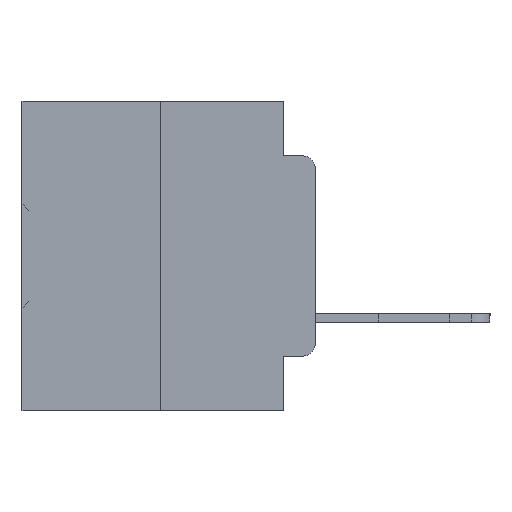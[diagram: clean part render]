
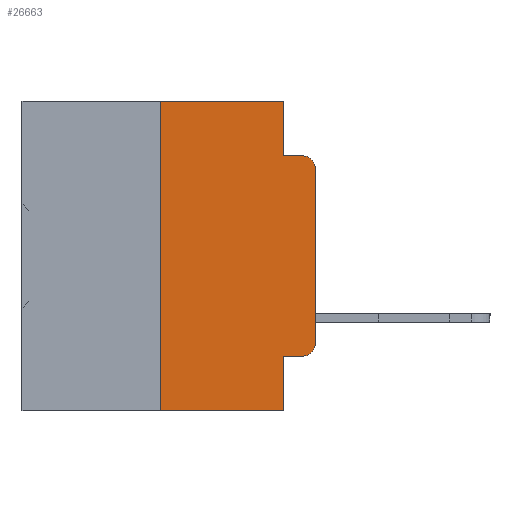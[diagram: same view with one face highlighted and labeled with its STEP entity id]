
A CAD part, left-side view. The second image highlights one B-rep face of the part: STEP entity #26663.
In plain terms, the highlighted planar face has unit normal (-1, 0, 0).
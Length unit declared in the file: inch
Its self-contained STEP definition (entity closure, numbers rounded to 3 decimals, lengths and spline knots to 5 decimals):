
#154 = DIRECTION ( 'NONE',  ( 0., 0., -1. ) ) ;
#941 = FACE_OUTER_BOUND ( 'NONE', #30080, .T. ) ;
#1112 = ORIENTED_EDGE ( 'NONE', *, *, #12248, .T. ) ;
#1768 = VERTEX_POINT ( 'NONE', #36380 ) ;
#2023 = DIRECTION ( 'NONE',  ( 0., 0., -1. ) ) ;
#2344 = LINE ( 'NONE', #2949, #23385 ) ;
#2350 = CARTESIAN_POINT ( 'NONE',  ( 0., 0.02, -0.4115 ) ) ;
#2720 = DIRECTION ( 'NONE',  ( 0., 0., -1. ) ) ;
#2949 = CARTESIAN_POINT ( 'NONE',  ( 0., 0.473, 0. ) ) ;
#2981 = VERTEX_POINT ( 'NONE', #11474 ) ;
#3852 = LINE ( 'NONE', #6824, #25783 ) ;
#5730 = EDGE_CURVE ( 'NONE', #36417, #1768, #3852, .T. ) ;
#5749 = CARTESIAN_POINT ( 'NONE',  ( 0., 0.25, -0.5 ) ) ;
#6105 = ORIENTED_EDGE ( 'NONE', *, *, #5730, .T. ) ;
#6185 = AXIS2_PLACEMENT_3D ( 'NONE', #30549, #13515, #33371 ) ;
#6299 = CARTESIAN_POINT ( 'NONE',  ( 0., 0.25, 0. ) ) ;
#6824 = CARTESIAN_POINT ( 'NONE',  ( 0., 0., 0. ) ) ;
#6929 = VERTEX_POINT ( 'NONE', #24255 ) ;
#7170 = LINE ( 'NONE', #9047, #21484 ) ;
#7693 = CARTESIAN_POINT ( 'NONE',  ( 0., 0.473, 0. ) ) ;
#7795 = CIRCLE ( 'NONE', #6185, 0.02 ) ;
#7893 = VECTOR ( 'NONE', #21350, 39.37008 ) ;
#8385 = CIRCLE ( 'NONE', #18694, 0.02 ) ;
#8658 = ORIENTED_EDGE ( 'NONE', *, *, #14152, .T. ) ;
#9005 = LINE ( 'NONE', #16842, #24184 ) ;
#9047 = CARTESIAN_POINT ( 'NONE',  ( 0., 0.051, -0.0885 ) ) ;
#9092 = DIRECTION ( 'NONE',  ( 0., 0., -1. ) ) ;
#9466 = LINE ( 'NONE', #34334, #23746 ) ;
#10687 = VECTOR ( 'NONE', #9092, 39.37008 ) ;
#11379 = AXIS2_PLACEMENT_3D ( 'NONE', #7693, #19181, #2023 ) ;
#11474 = CARTESIAN_POINT ( 'NONE',  ( 0., 0.02, -0.0885 ) ) ;
#11563 = ORIENTED_EDGE ( 'NONE', *, *, #29408, .F. ) ;
#11818 = VERTEX_POINT ( 'NONE', #5749 ) ;
#11909 = DIRECTION ( 'NONE',  ( 0., -1., 0. ) ) ;
#12248 = EDGE_CURVE ( 'NONE', #25647, #36417, #7795, .T. ) ;
#13139 = VERTEX_POINT ( 'NONE', #18095 ) ;
#13161 = CARTESIAN_POINT ( 'NONE',  ( 0., 0.473, -0.5 ) ) ;
#13515 = DIRECTION ( 'NONE',  ( -1., 0., 0. ) ) ;
#14152 = EDGE_CURVE ( 'NONE', #6929, #25647, #9005, .T. ) ;
#14358 = DIRECTION ( 'NONE',  ( 0., -1., 0. ) ) ;
#14693 = ORIENTED_EDGE ( 'NONE', *, *, #27518, .F. ) ;
#14969 = ORIENTED_EDGE ( 'NONE', *, *, #17990, .F. ) ;
#16077 = EDGE_CURVE ( 'NONE', #6929, #13139, #34216, .T. ) ;
#16516 = CARTESIAN_POINT ( 'NONE',  ( 0., 0.051, -0.0885 ) ) ;
#16829 = ORIENTED_EDGE ( 'NONE', *, *, #31294, .T. ) ;
#16842 = CARTESIAN_POINT ( 'NONE',  ( 0., 0.051, -0.4115 ) ) ;
#17990 = EDGE_CURVE ( 'NONE', #11818, #34008, #23089, .T. ) ;
#18095 = CARTESIAN_POINT ( 'NONE',  ( 0., 0.051, -0.5 ) ) ;
#18246 = VECTOR ( 'NONE', #27478, 39.37008 ) ;
#18498 = CARTESIAN_POINT ( 'NONE',  ( 0., 0.25, 0. ) ) ;
#18694 = AXIS2_PLACEMENT_3D ( 'NONE', #36735, #19896, #2720 ) ;
#19181 = DIRECTION ( 'NONE',  ( 1., 0., 0. ) ) ;
#19664 = CARTESIAN_POINT ( 'NONE',  ( 0., 0., -0.3915 ) ) ;
#19896 = DIRECTION ( 'NONE',  ( -1., 0., 0. ) ) ;
#20434 = CARTESIAN_POINT ( 'NONE',  ( 0., 0.051, 0. ) ) ;
#20657 = EDGE_CURVE ( 'NONE', #34008, #36102, #2344, .T. ) ;
#21350 = DIRECTION ( 'NONE',  ( 0., 0., 1. ) ) ;
#21484 = VECTOR ( 'NONE', #11909, 39.37008 ) ;
#21799 = CARTESIAN_POINT ( 'NONE',  ( 0., 0.051, 0. ) ) ;
#22240 = VERTEX_POINT ( 'NONE', #16516 ) ;
#22969 = ORIENTED_EDGE ( 'NONE', *, *, #20657, .F. ) ;
#23089 = LINE ( 'NONE', #18498, #7893 ) ;
#23385 = VECTOR ( 'NONE', #14358, 39.37008 ) ;
#23746 = VECTOR ( 'NONE', #154, 39.37008 ) ;
#23946 = ORIENTED_EDGE ( 'NONE', *, *, #16077, .F. ) ;
#23958 = DIRECTION ( 'NONE',  ( 0., 0., 1. ) ) ;
#24184 = VECTOR ( 'NONE', #36553, 39.37008 ) ;
#24255 = CARTESIAN_POINT ( 'NONE',  ( 0., 0.051, -0.4115 ) ) ;
#25647 = VERTEX_POINT ( 'NONE', #2350 ) ;
#25783 = VECTOR ( 'NONE', #23958, 39.37008 ) ;
#25813 = ORIENTED_EDGE ( 'NONE', *, *, #34825, .T. ) ;
#26663 = ADVANCED_FACE ( 'NONE', ( #941 ), #36080, .F. ) ;
#27478 = DIRECTION ( 'NONE',  ( 0., -1., 0. ) ) ;
#27518 = EDGE_CURVE ( 'NONE', #36102, #22240, #9466, .T. ) ;
#29408 = EDGE_CURVE ( 'NONE', #22240, #2981, #7170, .T. ) ;
#30080 = EDGE_LOOP ( 'NONE', ( #6105, #16829, #11563, #14693, #22969, #14969, #25813, #23946, #8658, #1112 ) ) ;
#30549 = CARTESIAN_POINT ( 'NONE',  ( 0., 0.02, -0.3915 ) ) ;
#31294 = EDGE_CURVE ( 'NONE', #1768, #2981, #8385, .T. ) ;
#33303 = LINE ( 'NONE', #13161, #18246 ) ;
#33371 = DIRECTION ( 'NONE',  ( 0., 0., -1. ) ) ;
#34008 = VERTEX_POINT ( 'NONE', #6299 ) ;
#34216 = LINE ( 'NONE', #20434, #10687 ) ;
#34334 = CARTESIAN_POINT ( 'NONE',  ( 0., 0.051, 0. ) ) ;
#34825 = EDGE_CURVE ( 'NONE', #11818, #13139, #33303, .T. ) ;
#36080 = PLANE ( 'NONE',  #11379 ) ;
#36102 = VERTEX_POINT ( 'NONE', #21799 ) ;
#36380 = CARTESIAN_POINT ( 'NONE',  ( 0., 0., -0.1085 ) ) ;
#36417 = VERTEX_POINT ( 'NONE', #19664 ) ;
#36553 = DIRECTION ( 'NONE',  ( 0., -1., 0. ) ) ;
#36735 = CARTESIAN_POINT ( 'NONE',  ( 0., 0.02, -0.1085 ) ) ;
